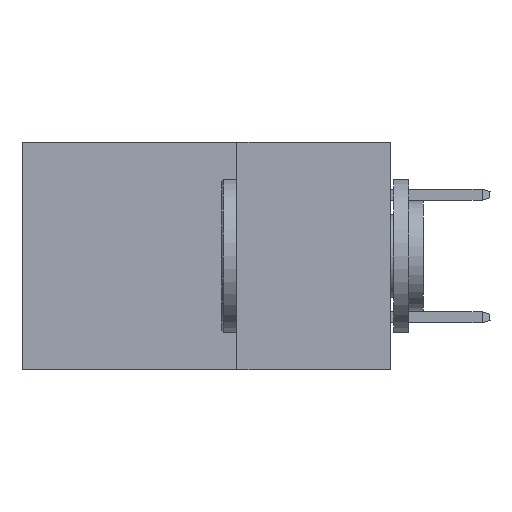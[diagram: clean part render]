
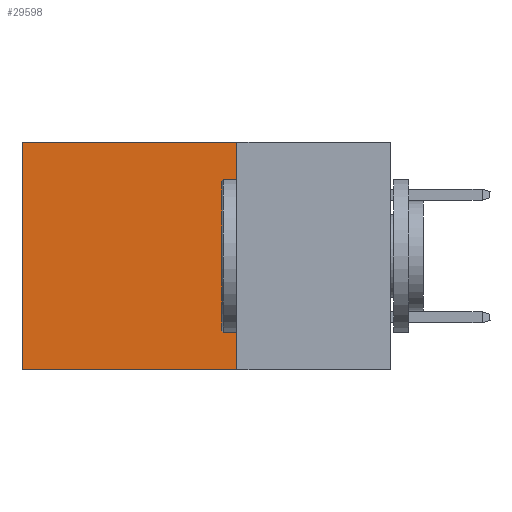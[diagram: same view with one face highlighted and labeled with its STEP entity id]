
A CAD part, left-side view. The second image highlights one B-rep face of the part: STEP entity #29598.
In plain terms, the highlighted planar face has unit normal (-1, 0, 0).
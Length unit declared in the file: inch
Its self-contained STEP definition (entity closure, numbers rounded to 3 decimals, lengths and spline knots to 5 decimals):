
#915 = EDGE_CURVE ( 'NONE', #20657, #29599, #12546, .T. ) ;
#1033 = VECTOR ( 'NONE', #1512, 39.37008 ) ;
#1415 = CARTESIAN_POINT ( 'NONE',  ( 0.2875, 0.25, 0. ) ) ;
#1512 = DIRECTION ( 'NONE',  ( 0., 1., 0. ) ) ;
#1879 = FACE_OUTER_BOUND ( 'NONE', #38620, .T. ) ;
#3015 = AXIS2_PLACEMENT_3D ( 'NONE', #37255, #19312, #28319 ) ;
#4437 = CARTESIAN_POINT ( 'NONE',  ( 0.2875, 0.25, -0.37 ) ) ;
#5438 = VECTOR ( 'NONE', #37286, 39.37008 ) ;
#6196 = LINE ( 'NONE', #4437, #1033 ) ;
#7042 = ORIENTED_EDGE ( 'NONE', *, *, #915, .T. ) ;
#7084 = LINE ( 'NONE', #14464, #38102 ) ;
#9756 = ORIENTED_EDGE ( 'NONE', *, *, #25129, .F. ) ;
#10347 = CARTESIAN_POINT ( 'NONE',  ( 0.2875, 0.6, 0. ) ) ;
#11575 = ORIENTED_EDGE ( 'NONE', *, *, #28391, .F. ) ;
#12546 = LINE ( 'NONE', #1415, #5438 ) ;
#13246 = CARTESIAN_POINT ( 'NONE',  ( 0.2875, 0.6, 0. ) ) ;
#13930 = EDGE_CURVE ( 'NONE', #29599, #22424, #35867, .T. ) ;
#14464 = CARTESIAN_POINT ( 'NONE',  ( 0.2875, 0.25, 0. ) ) ;
#14885 = ORIENTED_EDGE ( 'NONE', *, *, #13930, .T. ) ;
#15243 = DIRECTION ( 'NONE',  ( 0., 0., -1. ) ) ;
#15690 = VERTEX_POINT ( 'NONE', #29329 ) ;
#19312 = DIRECTION ( 'NONE',  ( 1., 0., 0. ) ) ;
#20657 = VERTEX_POINT ( 'NONE', #31128 ) ;
#22424 = VERTEX_POINT ( 'NONE', #33633 ) ;
#25129 = EDGE_CURVE ( 'NONE', #20657, #15690, #7084, .T. ) ;
#28214 = DIRECTION ( 'NONE',  ( 0., 0., -1. ) ) ;
#28319 = DIRECTION ( 'NONE',  ( 0., 0., -1. ) ) ;
#28391 = EDGE_CURVE ( 'NONE', #15690, #22424, #6196, .T. ) ;
#29329 = CARTESIAN_POINT ( 'NONE',  ( 0.2875, 0.25, -0.37 ) ) ;
#29598 = ADVANCED_FACE ( 'NONE', ( #1879 ), #31202, .F. ) ;
#29599 = VERTEX_POINT ( 'NONE', #10347 ) ;
#31128 = CARTESIAN_POINT ( 'NONE',  ( 0.2875, 0.25, 0. ) ) ;
#31202 = PLANE ( 'NONE',  #3015 ) ;
#33633 = CARTESIAN_POINT ( 'NONE',  ( 0.2875, 0.6, -0.37 ) ) ;
#34433 = VECTOR ( 'NONE', #28214, 39.37008 ) ;
#35867 = LINE ( 'NONE', #13246, #34433 ) ;
#37255 = CARTESIAN_POINT ( 'NONE',  ( 0.2875, 0.25, 0. ) ) ;
#37286 = DIRECTION ( 'NONE',  ( 0., 1., 0. ) ) ;
#38102 = VECTOR ( 'NONE', #15243, 39.37008 ) ;
#38620 = EDGE_LOOP ( 'NONE', ( #14885, #11575, #9756, #7042 ) ) ;
